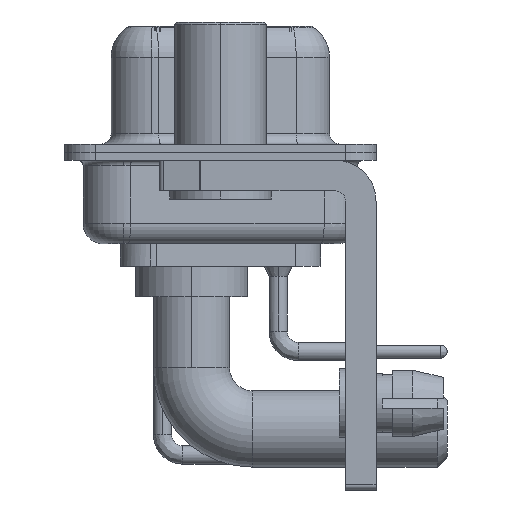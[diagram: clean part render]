
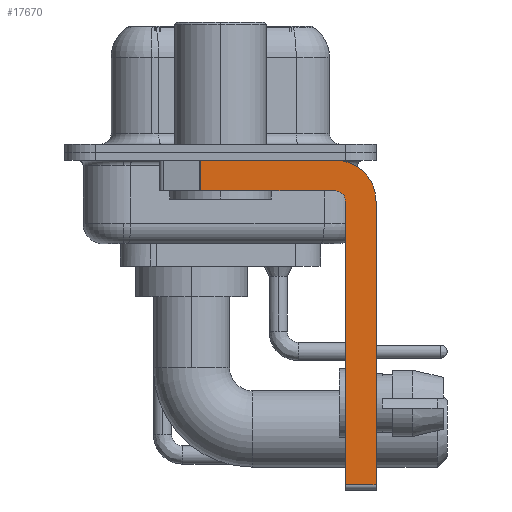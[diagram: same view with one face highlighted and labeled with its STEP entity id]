
A CAD part, left-side view. The second image highlights one B-rep face of the part: STEP entity #17670.
In plain terms, the highlighted planar face has unit normal (-1, 0, 0).
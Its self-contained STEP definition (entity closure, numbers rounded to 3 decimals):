
#489 = EDGE_CURVE ( 'NONE', #5818, #5970, #995, .T. ) ;
#995 = CIRCLE ( 'NONE', #26465, 2. ) ;
#1187 = VERTEX_POINT ( 'NONE', #11128 ) ;
#1320 = CARTESIAN_POINT ( 'NONE',  ( -2.9, -5.65, -2.4 ) ) ;
#2338 = VECTOR ( 'NONE', #6043, 1000. ) ;
#2898 = LINE ( 'NONE', #20338, #2338 ) ;
#3379 = DIRECTION ( 'NONE',  ( 0., 0., -1. ) ) ;
#3476 = FACE_OUTER_BOUND ( 'NONE', #22353, .T. ) ;
#3551 = ORIENTED_EDGE ( 'NONE', *, *, #36247, .T. ) ;
#3595 = EDGE_CURVE ( 'NONE', #11703, #5818, #2898, .T. ) ;
#4183 = EDGE_CURVE ( 'NONE', #1187, #23989, #9357, .T. ) ;
#4808 = VECTOR ( 'NONE', #13835, 1000. ) ;
#5025 = EDGE_CURVE ( 'NONE', #5970, #23172, #22418, .T. ) ;
#5438 = EDGE_CURVE ( 'NONE', #1187, #23172, #27902, .T. ) ;
#5669 = CARTESIAN_POINT ( 'NONE',  ( -2.9, 0.978, -0.4 ) ) ;
#5818 = VERTEX_POINT ( 'NONE', #27120 ) ;
#5970 = VERTEX_POINT ( 'NONE', #16756 ) ;
#6043 = DIRECTION ( 'NONE',  ( 0., -1., 0. ) ) ;
#6439 = ORIENTED_EDGE ( 'NONE', *, *, #489, .F. ) ;
#6544 = CARTESIAN_POINT ( 'NONE',  ( -2.9, 0.978, -1.9 ) ) ;
#7079 = DIRECTION ( 'NONE',  ( -1., 0., 0. ) ) ;
#7120 = CARTESIAN_POINT ( 'NONE',  ( -2.9, -6.15, -2.4 ) ) ;
#7333 = EDGE_CURVE ( 'NONE', #23989, #24295, #22011, .T. ) ;
#8293 = VECTOR ( 'NONE', #15301, 1000. ) ;
#8946 = ORIENTED_EDGE ( 'NONE', *, *, #27688, .F. ) ;
#9252 = DIRECTION ( 'NONE',  ( 1., 0., 0. ) ) ;
#9316 = AXIS2_PLACEMENT_3D ( 'NONE', #12044, #9252, #20556 ) ;
#9357 = LINE ( 'NONE', #26926, #8293 ) ;
#11128 = CARTESIAN_POINT ( 'NONE',  ( -2.9, -6.15, -16.35 ) ) ;
#11326 = CARTESIAN_POINT ( 'NONE',  ( -2.9, 0.978, -1.9 ) ) ;
#11691 = DIRECTION ( 'NONE',  ( 0., 0., -1. ) ) ;
#11703 = VERTEX_POINT ( 'NONE', #5669 ) ;
#12044 = CARTESIAN_POINT ( 'NONE',  ( -2.9, -5.65, -2.4 ) ) ;
#13835 = DIRECTION ( 'NONE',  ( 0., -1., 0. ) ) ;
#14690 = ORIENTED_EDGE ( 'NONE', *, *, #7333, .F. ) ;
#14829 = PLANE ( 'NONE',  #9316 ) ;
#15301 = DIRECTION ( 'NONE',  ( 0., 0., 1. ) ) ;
#15467 = VECTOR ( 'NONE', #11691, 1000. ) ;
#16756 = CARTESIAN_POINT ( 'NONE',  ( -2.9, -7.65, -2.4 ) ) ;
#17311 = CARTESIAN_POINT ( 'NONE',  ( -2.9, -5.65, -1.9 ) ) ;
#17333 = LINE ( 'NONE', #6544, #24041 ) ;
#17670 = ADVANCED_FACE ( 'NONE', ( #3476 ), #14829, .F. ) ;
#18173 = LINE ( 'NONE', #29453, #36114 ) ;
#20259 = AXIS2_PLACEMENT_3D ( 'NONE', #1320, #7079, #24312 ) ;
#20338 = CARTESIAN_POINT ( 'NONE',  ( -2.9, 3., -0.4 ) ) ;
#20556 = DIRECTION ( 'NONE',  ( 0., 0., -1. ) ) ;
#20695 = ORIENTED_EDGE ( 'NONE', *, *, #5025, .F. ) ;
#21114 = DIRECTION ( 'NONE',  ( 0., 1., 0. ) ) ;
#22011 = CIRCLE ( 'NONE', #20259, 0.5 ) ;
#22353 = EDGE_LOOP ( 'NONE', ( #32993, #3551, #8946, #14690, #26083, #26507, #20695, #6439 ) ) ;
#22418 = LINE ( 'NONE', #31337, #15467 ) ;
#23172 = VERTEX_POINT ( 'NONE', #34458 ) ;
#23989 = VERTEX_POINT ( 'NONE', #7120 ) ;
#24041 = VECTOR ( 'NONE', #3379, 1000. ) ;
#24295 = VERTEX_POINT ( 'NONE', #17311 ) ;
#24312 = DIRECTION ( 'NONE',  ( 0., 0., 1. ) ) ;
#26083 = ORIENTED_EDGE ( 'NONE', *, *, #4183, .F. ) ;
#26465 = AXIS2_PLACEMENT_3D ( 'NONE', #35726, #32951, #36639 ) ;
#26507 = ORIENTED_EDGE ( 'NONE', *, *, #5438, .T. ) ;
#26926 = CARTESIAN_POINT ( 'NONE',  ( -2.9, -6.15, -16.6 ) ) ;
#27120 = CARTESIAN_POINT ( 'NONE',  ( -2.9, -5.65, -0.4 ) ) ;
#27351 = CARTESIAN_POINT ( 'NONE',  ( -2.9, -5.65, -16.35 ) ) ;
#27688 = EDGE_CURVE ( 'NONE', #24295, #31728, #18173, .T. ) ;
#27902 = LINE ( 'NONE', #27351, #4808 ) ;
#29453 = CARTESIAN_POINT ( 'NONE',  ( -2.9, -5.65, -1.9 ) ) ;
#31337 = CARTESIAN_POINT ( 'NONE',  ( -2.9, -7.65, -2.4 ) ) ;
#31728 = VERTEX_POINT ( 'NONE', #11326 ) ;
#32951 = DIRECTION ( 'NONE',  ( 1., 0., 0. ) ) ;
#32993 = ORIENTED_EDGE ( 'NONE', *, *, #3595, .F. ) ;
#34458 = CARTESIAN_POINT ( 'NONE',  ( -2.9, -7.65, -16.35 ) ) ;
#35726 = CARTESIAN_POINT ( 'NONE',  ( -2.9, -5.65, -2.4 ) ) ;
#36114 = VECTOR ( 'NONE', #21114, 1000. ) ;
#36247 = EDGE_CURVE ( 'NONE', #11703, #31728, #17333, .T. ) ;
#36639 = DIRECTION ( 'NONE',  ( 0., 0., -1. ) ) ;
